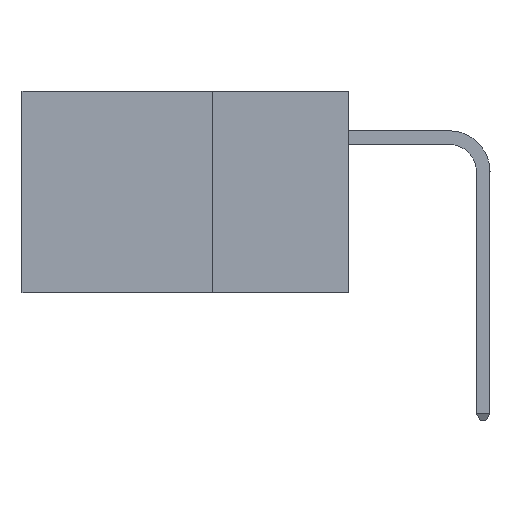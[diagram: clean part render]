
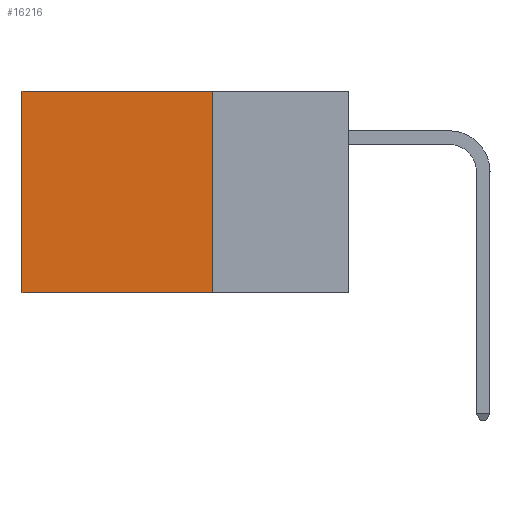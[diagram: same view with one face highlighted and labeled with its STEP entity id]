
A CAD part, left-side view. The second image highlights one B-rep face of the part: STEP entity #16216.
In plain terms, the highlighted planar face has unit normal (-1, 0, 0).
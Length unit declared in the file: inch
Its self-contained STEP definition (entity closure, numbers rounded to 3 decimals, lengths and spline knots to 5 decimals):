
#1473 = ORIENTED_EDGE ( 'NONE', *, *, #12372, .F. ) ;
#1722 = CARTESIAN_POINT ( 'NONE',  ( 0.2875, 0.25, 0. ) ) ;
#1757 = CARTESIAN_POINT ( 'NONE',  ( 0.2875, 0.6, 0. ) ) ;
#1895 = LINE ( 'NONE', #16581, #14254 ) ;
#4234 = CARTESIAN_POINT ( 'NONE',  ( 0.2875, 0.25, 0. ) ) ;
#5257 = CARTESIAN_POINT ( 'NONE',  ( 0.2875, 0.25, -0.37 ) ) ;
#5690 = CARTESIAN_POINT ( 'NONE',  ( 0.2875, 0.6, -0.37 ) ) ;
#6280 = VECTOR ( 'NONE', #8645, 39.37008 ) ;
#6788 = DIRECTION ( 'NONE',  ( 0., 1., 0. ) ) ;
#7217 = EDGE_CURVE ( 'NONE', #23447, #18105, #24734, .T. ) ;
#7242 = ORIENTED_EDGE ( 'NONE', *, *, #17849, .F. ) ;
#8492 = CARTESIAN_POINT ( 'NONE',  ( 0.2875, 0.25, 0. ) ) ;
#8645 = DIRECTION ( 'NONE',  ( 0., 0., -1. ) ) ;
#10182 = CARTESIAN_POINT ( 'NONE',  ( 0.2875, 0.6, 0. ) ) ;
#10549 = VERTEX_POINT ( 'NONE', #19554 ) ;
#11513 = PLANE ( 'NONE',  #16620 ) ;
#12202 = EDGE_CURVE ( 'NONE', #10549, #23447, #20933, .T. ) ;
#12372 = EDGE_CURVE ( 'NONE', #10549, #29683, #22585, .T. ) ;
#13583 = DIRECTION ( 'NONE',  ( 0., 1., 0. ) ) ;
#14254 = VECTOR ( 'NONE', #6788, 39.37008 ) ;
#16216 = ADVANCED_FACE ( 'NONE', ( #22704 ), #11513, .F. ) ;
#16581 = CARTESIAN_POINT ( 'NONE',  ( 0.2875, 0.25, -0.37 ) ) ;
#16620 = AXIS2_PLACEMENT_3D ( 'NONE', #1722, #30064, #27906 ) ;
#17800 = ORIENTED_EDGE ( 'NONE', *, *, #12202, .T. ) ;
#17849 = EDGE_CURVE ( 'NONE', #29683, #18105, #1895, .T. ) ;
#18105 = VERTEX_POINT ( 'NONE', #5690 ) ;
#19554 = CARTESIAN_POINT ( 'NONE',  ( 0.2875, 0.25, 0. ) ) ;
#20933 = LINE ( 'NONE', #4234, #22392 ) ;
#22392 = VECTOR ( 'NONE', #13583, 39.37008 ) ;
#22585 = LINE ( 'NONE', #8492, #6280 ) ;
#22586 = DIRECTION ( 'NONE',  ( 0., 0., -1. ) ) ;
#22704 = FACE_OUTER_BOUND ( 'NONE', #27880, .T. ) ;
#23447 = VERTEX_POINT ( 'NONE', #10182 ) ;
#24734 = LINE ( 'NONE', #1757, #26177 ) ;
#26177 = VECTOR ( 'NONE', #22586, 39.37008 ) ;
#26621 = ORIENTED_EDGE ( 'NONE', *, *, #7217, .T. ) ;
#27880 = EDGE_LOOP ( 'NONE', ( #26621, #7242, #1473, #17800 ) ) ;
#27906 = DIRECTION ( 'NONE',  ( 0., 0., -1. ) ) ;
#29683 = VERTEX_POINT ( 'NONE', #5257 ) ;
#30064 = DIRECTION ( 'NONE',  ( 1., 0., 0. ) ) ;
